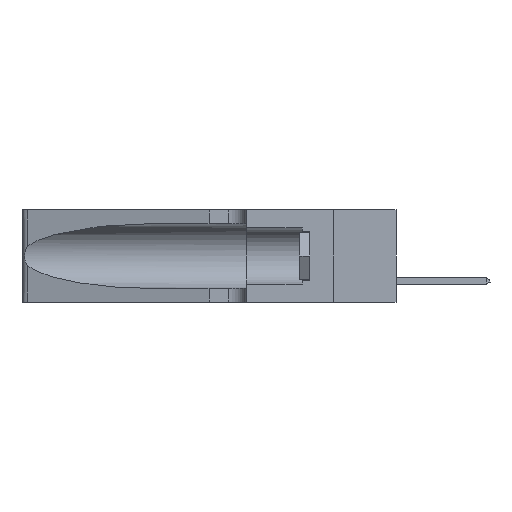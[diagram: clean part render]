
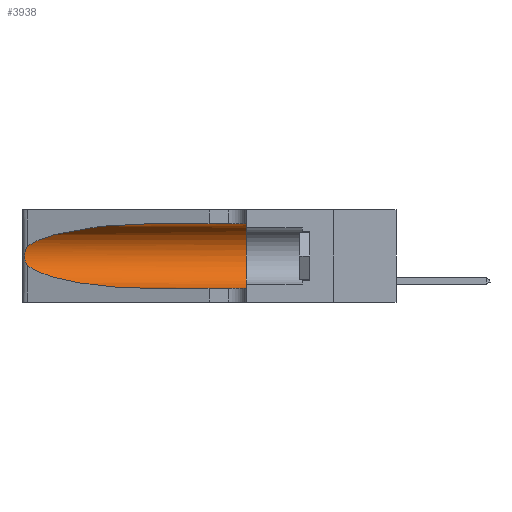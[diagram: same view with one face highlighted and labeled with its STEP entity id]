
A CAD part, left-side view. The second image highlights one B-rep face of the part: STEP entity #3938.
In plain terms, the highlighted cylindrical face has radius 3.308 mm (diameter 6.617 mm), a partial arc.
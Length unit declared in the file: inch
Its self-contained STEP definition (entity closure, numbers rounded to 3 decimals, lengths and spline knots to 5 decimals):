
#943 = CARTESIAN_POINT ( 'NONE',  ( 0.25555, 1.22994, 0.2215 ) ) ;
#1139 = CARTESIAN_POINT ( 'NONE',  ( 0.1305, 0.35, 0.185 ) ) ;
#1363 = VECTOR ( 'NONE', #13915, 39.37008 ) ;
#1489 = EDGE_CURVE ( 'NONE', #1688, #31782, #13528, .T. ) ;
#1534 = VERTEX_POINT ( 'NONE', #9362 ) ;
#1688 = VERTEX_POINT ( 'NONE', #25857 ) ;
#3805 = CARTESIAN_POINT ( 'NONE',  ( 0.25856, 1.23593, 0.16098 ) ) ;
#3932 = CARTESIAN_POINT ( 'NONE',  ( 0.26075, 1.23896, 0.178 ) ) ;
#3938 = ADVANCED_FACE ( 'NONE', ( #18271 ), #14495, .F. ) ;
#4065 = CARTESIAN_POINT ( 'NONE',  ( 0.26075, 1.23896, 0.19203 ) ) ;
#4815 = VERTEX_POINT ( 'NONE', #22948 ) ;
#5297 = VERTEX_POINT ( 'NONE', #8221 ) ;
#5361 = DIRECTION ( 'NONE',  ( 0., 0., -1. ) ) ;
#8015 = VECTOR ( 'NONE', #9563, 39.37008 ) ;
#8112 = EDGE_CURVE ( 'NONE', #1534, #5297, #8545, .T. ) ;
#8221 = CARTESIAN_POINT ( 'NONE',  ( 0.1305, 0.35, 0.31525 ) ) ;
#8267 = ORIENTED_EDGE ( 'NONE', *, *, #10129, .T. ) ;
#8545 = LINE ( 'NONE', #33118, #1363 ) ;
#9004 = CARTESIAN_POINT ( 'NONE',  ( 0.26018, 1.23835, 0.19895 ) ) ;
#9362 = CARTESIAN_POINT ( 'NONE',  ( 0.1305, 0.72297, 0.31525 ) ) ;
#9411 = ORIENTED_EDGE ( 'NONE', *, *, #17808, .T. ) ;
#9563 = DIRECTION ( 'NONE',  ( 0., -1., 0. ) ) ;
#10016 = CARTESIAN_POINT ( 'NONE',  ( 0.18966, 0.96281, 0.05475 ) ) ;
#10129 = EDGE_CURVE ( 'NONE', #1534, #1688, #12019, .T. ) ;
#11722 = CARTESIAN_POINT ( 'NONE',  ( 0.25789, 1.23486, 0.15765 ) ) ;
#12019 =( BOUNDED_CURVE ( )  B_SPLINE_CURVE ( 3, ( #18077, #26801, #13249, #29305 ),
 .UNSPECIFIED., .F., .T. ) 
 B_SPLINE_CURVE_WITH_KNOTS ( ( 4, 4 ),
 ( 1.5708, 2.84003 ),
 .UNSPECIFIED. ) 
 CURVE ( )  GEOMETRIC_REPRESENTATION_ITEM ( )  RATIONAL_B_SPLINE_CURVE ( ( 1., 0.87, 0.87, 1. ) ) 
 REPRESENTATION_ITEM ( '' )  );
#13249 = CARTESIAN_POINT ( 'NONE',  ( 0.2373, 1.15595, 0.28018 ) ) ;
#13528 = B_SPLINE_CURVE_WITH_KNOTS ( 'NONE', 3,
 ( #25262, #943, #14549, #22742, #20088, #9004, #4065, #3932, #19844, #3805, #11722, #33489, #20217, #33376 ),
 .UNSPECIFIED., .F., .F.,
 ( 4, 2, 2, 2, 2, 2, 4 ),
 ( 0., 0.00027, 0.00053, 0.00107, 0.0016, 0.00187, 0.00214 ),
 .UNSPECIFIED. ) ;
#13915 = DIRECTION ( 'NONE',  ( 0., -1., 0. ) ) ;
#14153 = VERTEX_POINT ( 'NONE', #14510 ) ;
#14495 = CYLINDRICAL_SURFACE ( 'NONE', #25681, 0.13025 ) ;
#14510 = CARTESIAN_POINT ( 'NONE',  ( 0.1305, 0.35, 0.05475 ) ) ;
#14549 = CARTESIAN_POINT ( 'NONE',  ( 0.25639, 1.23184, 0.21858 ) ) ;
#15382 =( BOUNDED_CURVE ( )  B_SPLINE_CURVE ( 3, ( #26397, #34472, #10016, #18005 ),
 .UNSPECIFIED., .F., .F. ) 
 B_SPLINE_CURVE_WITH_KNOTS ( ( 4, 4 ),
 ( 3.44316, 4.71239 ),
 .UNSPECIFIED. ) 
 CURVE ( )  GEOMETRIC_REPRESENTATION_ITEM ( )  RATIONAL_B_SPLINE_CURVE ( ( 1., 0.87, 0.87, 1. ) ) 
 REPRESENTATION_ITEM ( '' )  );
#15829 = CARTESIAN_POINT ( 'NONE',  ( 0.1305, 1.61858, 0.185 ) ) ;
#15938 = ORIENTED_EDGE ( 'NONE', *, *, #1489, .T. ) ;
#16845 = ORIENTED_EDGE ( 'NONE', *, *, #34072, .F. ) ;
#17808 = EDGE_CURVE ( 'NONE', #31782, #4815, #15382, .T. ) ;
#18005 = CARTESIAN_POINT ( 'NONE',  ( 0.1305, 0.72297, 0.05475 ) ) ;
#18011 = ORIENTED_EDGE ( 'NONE', *, *, #8112, .F. ) ;
#18077 = CARTESIAN_POINT ( 'NONE',  ( 0.1305, 0.72297, 0.31525 ) ) ;
#18271 = FACE_OUTER_BOUND ( 'NONE', #31416, .T. ) ;
#18425 = EDGE_CURVE ( 'NONE', #4815, #14153, #21977, .T. ) ;
#19844 = CARTESIAN_POINT ( 'NONE',  ( 0.26017, 1.23833, 0.17102 ) ) ;
#20088 = CARTESIAN_POINT ( 'NONE',  ( 0.25854, 1.2359, 0.20912 ) ) ;
#20217 = CARTESIAN_POINT ( 'NONE',  ( 0.25555, 1.22993, 0.14849 ) ) ;
#21722 = AXIS2_PLACEMENT_3D ( 'NONE', #1139, #33563, #22566 ) ;
#21977 = LINE ( 'NONE', #34052, #8015 ) ;
#22566 = DIRECTION ( 'NONE',  ( 0., 0., 1. ) ) ;
#22742 = CARTESIAN_POINT ( 'NONE',  ( 0.25787, 1.23484, 0.2124 ) ) ;
#22948 = CARTESIAN_POINT ( 'NONE',  ( 0.1305, 0.72297, 0.05475 ) ) ;
#25262 = CARTESIAN_POINT ( 'NONE',  ( 0.25487, 1.22718, 0.22369 ) ) ;
#25681 = AXIS2_PLACEMENT_3D ( 'NONE', #15829, #27011, #5361 ) ;
#25857 = CARTESIAN_POINT ( 'NONE',  ( 0.25487, 1.22718, 0.22369 ) ) ;
#26397 = CARTESIAN_POINT ( 'NONE',  ( 0.25487, 1.22718, 0.14631 ) ) ;
#26801 = CARTESIAN_POINT ( 'NONE',  ( 0.18966, 0.96281, 0.31525 ) ) ;
#27011 = DIRECTION ( 'NONE',  ( 0., -1., 0. ) ) ;
#28324 = CARTESIAN_POINT ( 'NONE',  ( 0.25487, 1.22718, 0.14631 ) ) ;
#29038 = CIRCLE ( 'NONE', #21722, 0.13025 ) ;
#29305 = CARTESIAN_POINT ( 'NONE',  ( 0.25487, 1.22718, 0.22369 ) ) ;
#31416 = EDGE_LOOP ( 'NONE', ( #8267, #15938, #9411, #31513, #16845, #18011 ) ) ;
#31513 = ORIENTED_EDGE ( 'NONE', *, *, #18425, .T. ) ;
#31782 = VERTEX_POINT ( 'NONE', #28324 ) ;
#33118 = CARTESIAN_POINT ( 'NONE',  ( 0.1305, 1.61858, 0.31525 ) ) ;
#33376 = CARTESIAN_POINT ( 'NONE',  ( 0.25487, 1.22718, 0.14631 ) ) ;
#33489 = CARTESIAN_POINT ( 'NONE',  ( 0.25639, 1.23186, 0.15144 ) ) ;
#33563 = DIRECTION ( 'NONE',  ( 0., 1., 0. ) ) ;
#34052 = CARTESIAN_POINT ( 'NONE',  ( 0.1305, 1.61858, 0.05475 ) ) ;
#34072 = EDGE_CURVE ( 'NONE', #5297, #14153, #29038, .T. ) ;
#34472 = CARTESIAN_POINT ( 'NONE',  ( 0.2373, 1.15595, 0.08982 ) ) ;
